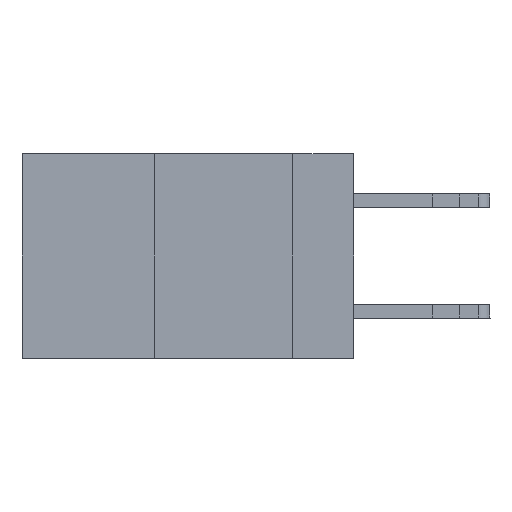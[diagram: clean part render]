
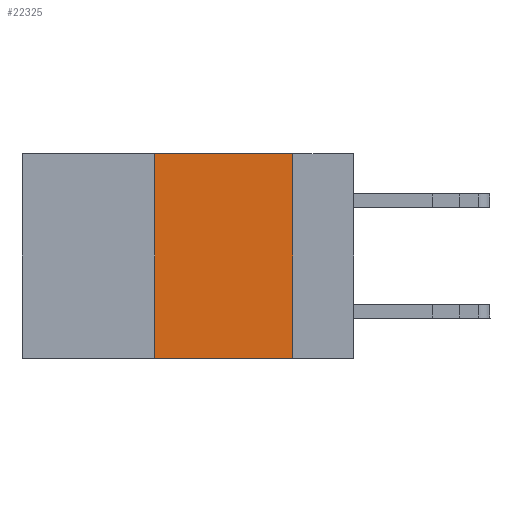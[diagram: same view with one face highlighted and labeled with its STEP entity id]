
A CAD part, left-side view. The second image highlights one B-rep face of the part: STEP entity #22325.
In plain terms, the highlighted planar face has unit normal (-1, 0, 0).
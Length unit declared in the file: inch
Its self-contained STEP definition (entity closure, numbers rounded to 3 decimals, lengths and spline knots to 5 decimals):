
#174 = VECTOR ( 'NONE', #401, 39.37008 ) ;
#401 = DIRECTION ( 'NONE',  ( 0., -1., 0. ) ) ;
#831 = FACE_OUTER_BOUND ( 'NONE', #20581, .T. ) ;
#947 = DIRECTION ( 'NONE',  ( 0., 0., -1. ) ) ;
#969 = CARTESIAN_POINT ( 'NONE',  ( 0., 0.36, -0.37 ) ) ;
#1377 = LINE ( 'NONE', #20297, #21549 ) ;
#1612 = DIRECTION ( 'NONE',  ( 0., -1., 0. ) ) ;
#2022 = EDGE_CURVE ( 'NONE', #20465, #23819, #18118, .T. ) ;
#2353 = ORIENTED_EDGE ( 'NONE', *, *, #17194, .F. ) ;
#2798 = CARTESIAN_POINT ( 'NONE',  ( 0., 0.11, 0. ) ) ;
#3539 = CARTESIAN_POINT ( 'NONE',  ( 0., 0.11, -0.37 ) ) ;
#4370 = EDGE_CURVE ( 'NONE', #16036, #23819, #1377, .T. ) ;
#4560 = PLANE ( 'NONE',  #18271 ) ;
#5760 = LINE ( 'NONE', #13357, #174 ) ;
#6205 = CARTESIAN_POINT ( 'NONE',  ( 0., 0.36, 0. ) ) ;
#7593 = ORIENTED_EDGE ( 'NONE', *, *, #11017, .F. ) ;
#8190 = DIRECTION ( 'NONE',  ( 0., 0., -1. ) ) ;
#9925 = LINE ( 'NONE', #6205, #22320 ) ;
#10011 = ORIENTED_EDGE ( 'NONE', *, *, #2022, .F. ) ;
#11017 = EDGE_CURVE ( 'NONE', #22029, #20465, #5760, .T. ) ;
#11810 = DIRECTION ( 'NONE',  ( 0., 0., 1. ) ) ;
#13357 = CARTESIAN_POINT ( 'NONE',  ( 0., 0.6, 0. ) ) ;
#14394 = CARTESIAN_POINT ( 'NONE',  ( 0., 0.6, 0. ) ) ;
#14796 = CARTESIAN_POINT ( 'NONE',  ( 0., 0.36, 0. ) ) ;
#16036 = VERTEX_POINT ( 'NONE', #969 ) ;
#17194 = EDGE_CURVE ( 'NONE', #16036, #22029, #9925, .T. ) ;
#17211 = CARTESIAN_POINT ( 'NONE',  ( 0., 0.11, 0. ) ) ;
#17303 = ORIENTED_EDGE ( 'NONE', *, *, #4370, .T. ) ;
#18118 = LINE ( 'NONE', #2798, #19052 ) ;
#18271 = AXIS2_PLACEMENT_3D ( 'NONE', #14394, #21996, #8190 ) ;
#19052 = VECTOR ( 'NONE', #947, 39.37008 ) ;
#20297 = CARTESIAN_POINT ( 'NONE',  ( 0., 0.6, -0.37 ) ) ;
#20465 = VERTEX_POINT ( 'NONE', #17211 ) ;
#20581 = EDGE_LOOP ( 'NONE', ( #10011, #7593, #2353, #17303 ) ) ;
#21549 = VECTOR ( 'NONE', #1612, 39.37008 ) ;
#21996 = DIRECTION ( 'NONE',  ( 1., 0., 0. ) ) ;
#22029 = VERTEX_POINT ( 'NONE', #14796 ) ;
#22320 = VECTOR ( 'NONE', #11810, 39.37008 ) ;
#22325 = ADVANCED_FACE ( 'NONE', ( #831 ), #4560, .F. ) ;
#23819 = VERTEX_POINT ( 'NONE', #3539 ) ;
